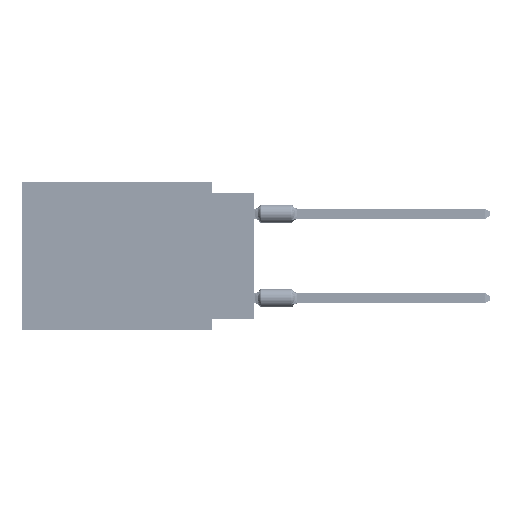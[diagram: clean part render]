
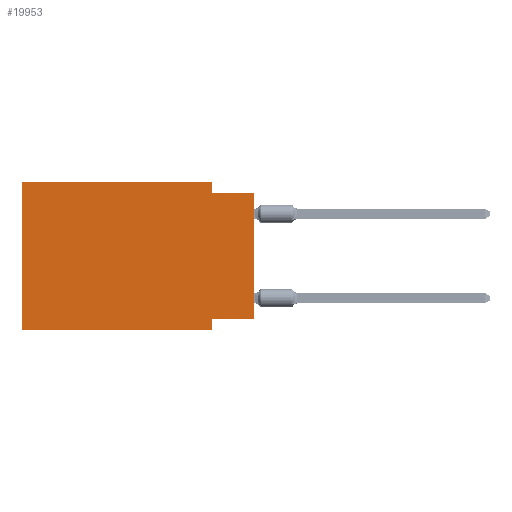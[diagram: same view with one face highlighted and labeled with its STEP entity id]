
A CAD part, left-side view. The second image highlights one B-rep face of the part: STEP entity #19953.
In plain terms, the highlighted planar face has unit normal (-1, 0, 0).
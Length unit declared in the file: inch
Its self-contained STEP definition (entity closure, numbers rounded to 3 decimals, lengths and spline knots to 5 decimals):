
#1708 = VECTOR ( 'NONE', #56921, 39.37008 ) ;
#5705 = DIRECTION ( 'NONE',  ( 0., 0., -1. ) ) ;
#6229 = DIRECTION ( 'NONE',  ( 0., 0., 1. ) ) ;
#6648 = VERTEX_POINT ( 'NONE', #62606 ) ;
#6722 = DIRECTION ( 'NONE',  ( 0., -1., 0. ) ) ;
#7218 = EDGE_CURVE ( 'NONE', #92658, #97450, #86788, .T. ) ;
#7547 = EDGE_CURVE ( 'NONE', #78874, #97450, #55279, .T. ) ;
#9876 = ORIENTED_EDGE ( 'NONE', *, *, #59351, .F. ) ;
#11264 = EDGE_CURVE ( 'NONE', #86949, #78874, #92388, .T. ) ;
#12299 = CARTESIAN_POINT ( 'NONE',  ( 0., 0.1, 0. ) ) ;
#13596 = DIRECTION ( 'NONE',  ( 1., 0., 0. ) ) ;
#13902 = EDGE_LOOP ( 'NONE', ( #79728, #91441, #9876, #91334, #21998, #49564, #92061, #34569 ) ) ;
#15906 = EDGE_CURVE ( 'NONE', #86949, #84025, #86406, .T. ) ;
#16810 = DIRECTION ( 'NONE',  ( 0., 0., -1. ) ) ;
#18328 = CARTESIAN_POINT ( 'NONE',  ( 0., 0.1, -0.35 ) ) ;
#18576 = VECTOR ( 'NONE', #5705, 39.37008 ) ;
#19953 = ADVANCED_FACE ( 'NONE', ( #59664 ), #74357, .F. ) ;
#20263 = CARTESIAN_POINT ( 'NONE',  ( 0., 0.1, -0.025 ) ) ;
#21998 = ORIENTED_EDGE ( 'NONE', *, *, #25506, .F. ) ;
#25506 = EDGE_CURVE ( 'NONE', #92658, #75009, #83662, .T. ) ;
#30314 = EDGE_CURVE ( 'NONE', #75009, #6648, #91257, .T. ) ;
#33059 = VECTOR ( 'NONE', #77182, 39.37008 ) ;
#34569 = ORIENTED_EDGE ( 'NONE', *, *, #11264, .F. ) ;
#40206 = CARTESIAN_POINT ( 'NONE',  ( 0., 0.55, -0.35 ) ) ;
#42643 = VECTOR ( 'NONE', #44139, 39.37008 ) ;
#44139 = DIRECTION ( 'NONE',  ( 0., -1., 0. ) ) ;
#44460 = DIRECTION ( 'NONE',  ( 0., 0., -1. ) ) ;
#45888 = VERTEX_POINT ( 'NONE', #20263 ) ;
#47928 = CARTESIAN_POINT ( 'NONE',  ( 0., 0., 0. ) ) ;
#49564 = ORIENTED_EDGE ( 'NONE', *, *, #7218, .T. ) ;
#49738 = CARTESIAN_POINT ( 'NONE',  ( 0., 0., -0.325 ) ) ;
#51746 = LINE ( 'NONE', #12299, #18576 ) ;
#55279 = LINE ( 'NONE', #18328, #85875 ) ;
#56921 = DIRECTION ( 'NONE',  ( 0., -1., 0. ) ) ;
#58090 = EDGE_CURVE ( 'NONE', #45888, #84025, #90716, .T. ) ;
#59351 = EDGE_CURVE ( 'NONE', #6648, #45888, #51746, .T. ) ;
#59664 = FACE_OUTER_BOUND ( 'NONE', #13902, .T. ) ;
#62009 = CARTESIAN_POINT ( 'NONE',  ( 0., 0., -0.325 ) ) ;
#62606 = CARTESIAN_POINT ( 'NONE',  ( 0., 0.1, 0. ) ) ;
#66512 = CARTESIAN_POINT ( 'NONE',  ( 0., 0.55, 0. ) ) ;
#69031 = VECTOR ( 'NONE', #6229, 39.37008 ) ;
#72285 = CARTESIAN_POINT ( 'NONE',  ( 0., 0.55, 0. ) ) ;
#73868 = CARTESIAN_POINT ( 'NONE',  ( 0., 0.55, 0. ) ) ;
#74357 = PLANE ( 'NONE',  #99191 ) ;
#75009 = VERTEX_POINT ( 'NONE', #72285 ) ;
#75450 = VECTOR ( 'NONE', #87914, 39.37008 ) ;
#75517 = CARTESIAN_POINT ( 'NONE',  ( 0., 0., -0.025 ) ) ;
#76737 = CARTESIAN_POINT ( 'NONE',  ( 0., 0.1, -0.35 ) ) ;
#77182 = DIRECTION ( 'NONE',  ( 0., 1., 0. ) ) ;
#78259 = CARTESIAN_POINT ( 'NONE',  ( 0., 0.1, -0.325 ) ) ;
#78874 = VERTEX_POINT ( 'NONE', #78259 ) ;
#79728 = ORIENTED_EDGE ( 'NONE', *, *, #15906, .T. ) ;
#80205 = CARTESIAN_POINT ( 'NONE',  ( 0., 0.55, -0.35 ) ) ;
#83662 = LINE ( 'NONE', #66512, #69031 ) ;
#84025 = VERTEX_POINT ( 'NONE', #85181 ) ;
#85181 = CARTESIAN_POINT ( 'NONE',  ( 0., 0., -0.025 ) ) ;
#85875 = VECTOR ( 'NONE', #16810, 39.37008 ) ;
#86406 = LINE ( 'NONE', #47928, #75450 ) ;
#86788 = LINE ( 'NONE', #40206, #1708 ) ;
#86949 = VERTEX_POINT ( 'NONE', #49738 ) ;
#87914 = DIRECTION ( 'NONE',  ( 0., 0., 1. ) ) ;
#88862 = VECTOR ( 'NONE', #6722, 39.37008 ) ;
#90716 = LINE ( 'NONE', #75517, #42643 ) ;
#90757 = CARTESIAN_POINT ( 'NONE',  ( 0., 0.55, 0. ) ) ;
#91257 = LINE ( 'NONE', #90757, #88862 ) ;
#91334 = ORIENTED_EDGE ( 'NONE', *, *, #30314, .F. ) ;
#91441 = ORIENTED_EDGE ( 'NONE', *, *, #58090, .F. ) ;
#92061 = ORIENTED_EDGE ( 'NONE', *, *, #7547, .F. ) ;
#92388 = LINE ( 'NONE', #62009, #33059 ) ;
#92658 = VERTEX_POINT ( 'NONE', #80205 ) ;
#97450 = VERTEX_POINT ( 'NONE', #76737 ) ;
#99191 = AXIS2_PLACEMENT_3D ( 'NONE', #73868, #13596, #44460 ) ;
